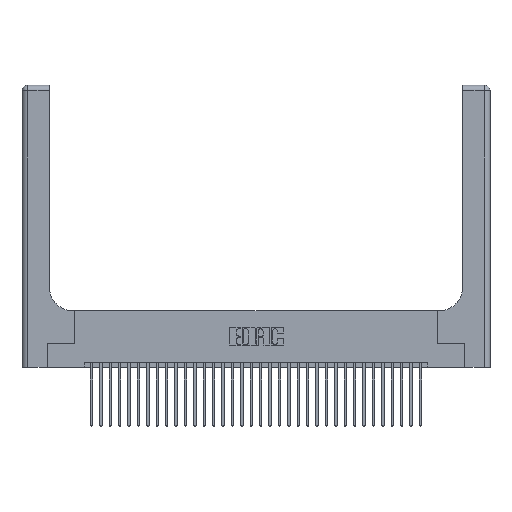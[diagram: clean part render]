
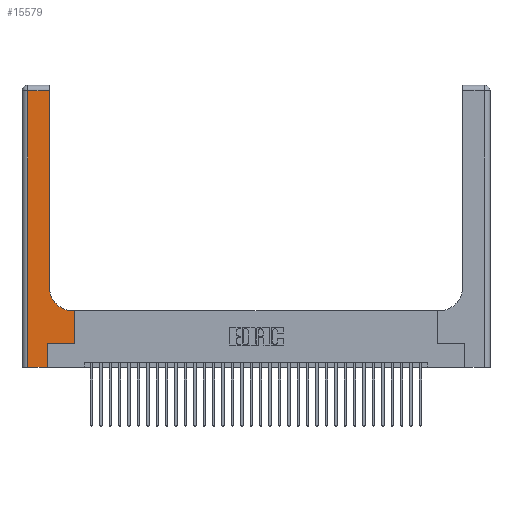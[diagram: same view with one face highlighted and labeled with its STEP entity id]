
A CAD part, top view. The second image highlights one B-rep face of the part: STEP entity #15579.
In plain terms, the highlighted planar face has unit normal (0, 0, 1).
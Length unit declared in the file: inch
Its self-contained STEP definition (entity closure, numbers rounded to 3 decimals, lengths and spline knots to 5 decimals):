
#148 = CARTESIAN_POINT ( 'NONE',  ( 0.269, 0.25, 0.37 ) ) ;
#264 = ORIENTED_EDGE ( 'NONE', *, *, #17795, .T. ) ;
#1047 = EDGE_CURVE ( 'NONE', #30656, #33497, #31131, .T. ) ;
#1223 = PLANE ( 'NONE',  #18676 ) ;
#2117 = CARTESIAN_POINT ( 'NONE',  ( 0.06, 3., 0.37 ) ) ;
#2536 = ORIENTED_EDGE ( 'NONE', *, *, #20774, .T. ) ;
#2713 = VECTOR ( 'NONE', #10015, 39.37008 ) ;
#4450 = CARTESIAN_POINT ( 'NONE',  ( 0.2915, 3., 0.37 ) ) ;
#4732 = CARTESIAN_POINT ( 'NONE',  ( 0.06, 2.94, 0.37 ) ) ;
#6288 = ORIENTED_EDGE ( 'NONE', *, *, #9754, .T. ) ;
#6997 = LINE ( 'NONE', #31363, #27233 ) ;
#7217 = VERTEX_POINT ( 'NONE', #17904 ) ;
#7427 = VERTEX_POINT ( 'NONE', #4732 ) ;
#7460 = CARTESIAN_POINT ( 'NONE',  ( 0.5585, 0.25, 0.37 ) ) ;
#7759 = LINE ( 'NONE', #14865, #26338 ) ;
#8174 = ORIENTED_EDGE ( 'NONE', *, *, #1047, .T. ) ;
#9295 = CARTESIAN_POINT ( 'NONE',  ( 0.5415, 0.85, 0.37 ) ) ;
#9754 = EDGE_CURVE ( 'NONE', #7427, #30656, #24833, .T. ) ;
#10015 = DIRECTION ( 'NONE',  ( 0., 1., 0. ) ) ;
#10703 = ORIENTED_EDGE ( 'NONE', *, *, #28659, .T. ) ;
#10979 = EDGE_CURVE ( 'NONE', #32538, #22873, #30993, .T. ) ;
#11108 = CARTESIAN_POINT ( 'NONE',  ( 0.2915, 0.85, 0.37 ) ) ;
#11426 = VECTOR ( 'NONE', #24111, 39.37008 ) ;
#11469 = CARTESIAN_POINT ( 'NONE',  ( 0., 3., 0.37 ) ) ;
#11494 = EDGE_CURVE ( 'NONE', #29360, #7217, #23044, .T. ) ;
#11693 = DIRECTION ( 'NONE',  ( -1., 0., 0. ) ) ;
#11975 = VECTOR ( 'NONE', #22741, 39.37008 ) ;
#14316 = VECTOR ( 'NONE', #31976, 39.37008 ) ;
#14865 = CARTESIAN_POINT ( 'NONE',  ( 0., 2.94, 0.37 ) ) ;
#15579 = ADVANCED_FACE ( 'NONE', ( #29680 ), #1223, .F. ) ;
#16451 = VECTOR ( 'NONE', #30865, 39.37008 ) ;
#16768 = AXIS2_PLACEMENT_3D ( 'NONE', #9295, #30482, #21289 ) ;
#17022 = DIRECTION ( 'NONE',  ( 0., 0., -1. ) ) ;
#17619 = LINE ( 'NONE', #148, #14316 ) ;
#17683 = CARTESIAN_POINT ( 'NONE',  ( 0., 0., 0.37 ) ) ;
#17795 = EDGE_CURVE ( 'NONE', #22873, #30138, #20482, .T. ) ;
#17904 = CARTESIAN_POINT ( 'NONE',  ( 0.5585, 0.6, 0.37 ) ) ;
#18154 = DIRECTION ( 'NONE',  ( -1., 0., 0. ) ) ;
#18676 = AXIS2_PLACEMENT_3D ( 'NONE', #11469, #17022, #11693 ) ;
#19698 = EDGE_CURVE ( 'NONE', #7217, #32538, #6997, .T. ) ;
#20028 = CARTESIAN_POINT ( 'NONE',  ( 0.269, 0., 0.37 ) ) ;
#20482 = LINE ( 'NONE', #4450, #2713 ) ;
#20774 = EDGE_CURVE ( 'NONE', #30138, #7427, #7759, .T. ) ;
#21289 = DIRECTION ( 'NONE',  ( 1., 0., 0. ) ) ;
#22741 = DIRECTION ( 'NONE',  ( 0., -1., 0. ) ) ;
#22873 = VERTEX_POINT ( 'NONE', #11108 ) ;
#22900 = DIRECTION ( 'NONE',  ( -1., 0., 0. ) ) ;
#23044 = LINE ( 'NONE', #23882, #11426 ) ;
#23384 = CARTESIAN_POINT ( 'NONE',  ( 0.269, 0.25, 0.37 ) ) ;
#23627 = ORIENTED_EDGE ( 'NONE', *, *, #31022, .T. ) ;
#23882 = CARTESIAN_POINT ( 'NONE',  ( 0.5585, 0.25, 0.37 ) ) ;
#24111 = DIRECTION ( 'NONE',  ( 0., 1., 0. ) ) ;
#24833 = LINE ( 'NONE', #2117, #11975 ) ;
#26338 = VECTOR ( 'NONE', #22900, 39.37008 ) ;
#26812 = CARTESIAN_POINT ( 'NONE',  ( 0.5415, 0.6, 0.37 ) ) ;
#26962 = ORIENTED_EDGE ( 'NONE', *, *, #10979, .T. ) ;
#27233 = VECTOR ( 'NONE', #18154, 39.37008 ) ;
#28364 = DIRECTION ( 'NONE',  ( 1., 0., 0. ) ) ;
#28659 = EDGE_CURVE ( 'NONE', #33497, #31462, #32216, .T. ) ;
#28711 = CARTESIAN_POINT ( 'NONE',  ( 0.06, 0., 0.37 ) ) ;
#29125 = CARTESIAN_POINT ( 'NONE',  ( 0.2915, 2.94, 0.37 ) ) ;
#29360 = VERTEX_POINT ( 'NONE', #7460 ) ;
#29680 = FACE_OUTER_BOUND ( 'NONE', #33758, .T. ) ;
#30138 = VERTEX_POINT ( 'NONE', #29125 ) ;
#30482 = DIRECTION ( 'NONE',  ( 0., 0., -1. ) ) ;
#30630 = ORIENTED_EDGE ( 'NONE', *, *, #19698, .T. ) ;
#30656 = VERTEX_POINT ( 'NONE', #28711 ) ;
#30749 = CARTESIAN_POINT ( 'NONE',  ( 0.269, 0., 0.37 ) ) ;
#30865 = DIRECTION ( 'NONE',  ( 0., 1., 0. ) ) ;
#30993 = CIRCLE ( 'NONE', #16768, 0.25 ) ;
#31022 = EDGE_CURVE ( 'NONE', #31462, #29360, #17619, .T. ) ;
#31131 = LINE ( 'NONE', #17683, #33175 ) ;
#31363 = CARTESIAN_POINT ( 'NONE',  ( 0.2915, 0.6, 0.37 ) ) ;
#31462 = VERTEX_POINT ( 'NONE', #23384 ) ;
#31976 = DIRECTION ( 'NONE',  ( 1., 0., 0. ) ) ;
#32216 = LINE ( 'NONE', #30749, #16451 ) ;
#32538 = VERTEX_POINT ( 'NONE', #26812 ) ;
#33175 = VECTOR ( 'NONE', #28364, 39.37008 ) ;
#33497 = VERTEX_POINT ( 'NONE', #20028 ) ;
#33758 = EDGE_LOOP ( 'NONE', ( #264, #2536, #6288, #8174, #10703, #23627, #33933, #30630, #26962 ) ) ;
#33933 = ORIENTED_EDGE ( 'NONE', *, *, #11494, .T. ) ;
